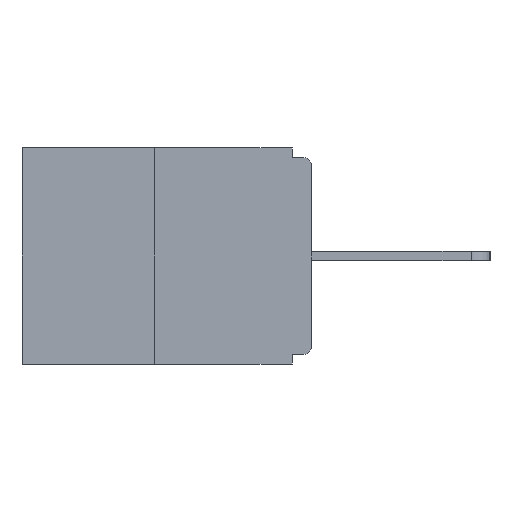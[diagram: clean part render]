
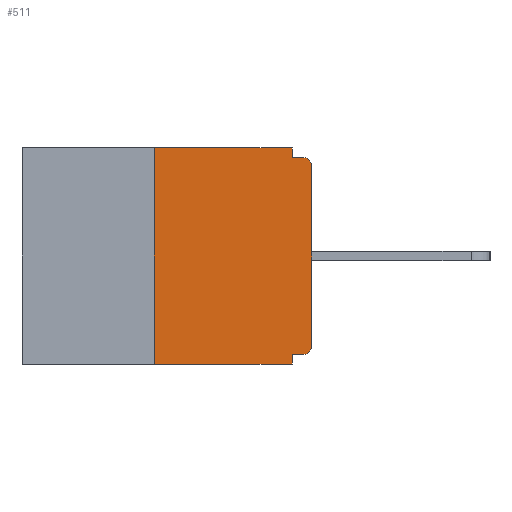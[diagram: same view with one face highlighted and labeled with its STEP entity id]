
A CAD part, left-side view. The second image highlights one B-rep face of the part: STEP entity #511.
In plain terms, the highlighted planar face has unit normal (-1, 0, 0).
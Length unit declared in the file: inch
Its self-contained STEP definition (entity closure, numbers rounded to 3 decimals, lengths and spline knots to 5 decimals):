
#488 = VECTOR ( 'NONE', #17203, 39.37008 ) ;
#509 = DIRECTION ( 'NONE',  ( 0., 0., 1. ) ) ;
#511 = ADVANCED_FACE ( 'NONE', ( #11315 ), #3797, .F. ) ;
#588 = CARTESIAN_POINT ( 'NONE',  ( 0., 0., 0. ) ) ;
#759 = DIRECTION ( 'NONE',  ( 1., 0., 0. ) ) ;
#874 = DIRECTION ( 'NONE',  ( 0., -1., 0. ) ) ;
#1120 = EDGE_LOOP ( 'NONE', ( #9245, #10424, #9022, #7291, #12049, #1280, #16525, #9086, #8726, #9004 ) ) ;
#1280 = ORIENTED_EDGE ( 'NONE', *, *, #3385, .T. ) ;
#1300 = VECTOR ( 'NONE', #509, 39.37008 ) ;
#1647 = VERTEX_POINT ( 'NONE', #1875 ) ;
#1843 = DIRECTION ( 'NONE',  ( 0., -1., 0. ) ) ;
#1875 = CARTESIAN_POINT ( 'NONE',  ( 0., 0., -0.03 ) ) ;
#2244 = CARTESIAN_POINT ( 'NONE',  ( 0., 0.25, 0. ) ) ;
#2885 = CARTESIAN_POINT ( 'NONE',  ( 0., 0.015, -0.03 ) ) ;
#2975 = CARTESIAN_POINT ( 'NONE',  ( 0., 0.031, -0.015 ) ) ;
#3385 = EDGE_CURVE ( 'NONE', #7476, #16054, #7079, .T. ) ;
#3548 = EDGE_CURVE ( 'NONE', #16054, #1647, #18411, .T. ) ;
#3797 = PLANE ( 'NONE',  #12862 ) ;
#3869 = LINE ( 'NONE', #6156, #15055 ) ;
#4214 = DIRECTION ( 'NONE',  ( -1., 0., 0. ) ) ;
#4341 = EDGE_CURVE ( 'NONE', #9982, #6168, #6028, .T. ) ;
#4819 = AXIS2_PLACEMENT_3D ( 'NONE', #2885, #10698, #16344 ) ;
#5270 = DIRECTION ( 'NONE',  ( 0., 0., -1. ) ) ;
#5628 = CARTESIAN_POINT ( 'NONE',  ( 0., 0.46, 0. ) ) ;
#6028 = LINE ( 'NONE', #5628, #488 ) ;
#6156 = CARTESIAN_POINT ( 'NONE',  ( 0., 0.031, -0.343 ) ) ;
#6168 = VERTEX_POINT ( 'NONE', #12745 ) ;
#6912 = CARTESIAN_POINT ( 'NONE',  ( 0., 0., -0.328 ) ) ;
#7079 = CIRCLE ( 'NONE', #17907, 0.015 ) ;
#7291 = ORIENTED_EDGE ( 'NONE', *, *, #10679, .F. ) ;
#7476 = VERTEX_POINT ( 'NONE', #11408 ) ;
#7525 = VECTOR ( 'NONE', #9132, 39.37008 ) ;
#8483 = CARTESIAN_POINT ( 'NONE',  ( 0., 0.015, -0.015 ) ) ;
#8532 = EDGE_CURVE ( 'NONE', #17141, #13712, #15683, .T. ) ;
#8726 = ORIENTED_EDGE ( 'NONE', *, *, #8532, .F. ) ;
#9004 = ORIENTED_EDGE ( 'NONE', *, *, #15616, .F. ) ;
#9014 = VERTEX_POINT ( 'NONE', #18674 ) ;
#9022 = ORIENTED_EDGE ( 'NONE', *, *, #18537, .T. ) ;
#9086 = ORIENTED_EDGE ( 'NONE', *, *, #9792, .T. ) ;
#9132 = DIRECTION ( 'NONE',  ( 0., 0., 1. ) ) ;
#9245 = ORIENTED_EDGE ( 'NONE', *, *, #4341, .F. ) ;
#9532 = CARTESIAN_POINT ( 'NONE',  ( 0., 0., -0.015 ) ) ;
#9620 = VERTEX_POINT ( 'NONE', #10843 ) ;
#9792 = EDGE_CURVE ( 'NONE', #1647, #13712, #12235, .T. ) ;
#9847 = DIRECTION ( 'NONE',  ( 0., 1., 0. ) ) ;
#9982 = VERTEX_POINT ( 'NONE', #13771 ) ;
#10038 = CARTESIAN_POINT ( 'NONE',  ( 0., 0.015, -0.313 ) ) ;
#10086 = EDGE_CURVE ( 'NONE', #7476, #9014, #17677, .T. ) ;
#10424 = ORIENTED_EDGE ( 'NONE', *, *, #15927, .F. ) ;
#10634 = CARTESIAN_POINT ( 'NONE',  ( 0., 0.031, 0. ) ) ;
#10679 = EDGE_CURVE ( 'NONE', #9014, #9620, #3869, .T. ) ;
#10698 = DIRECTION ( 'NONE',  ( -1., 0., 0. ) ) ;
#10843 = CARTESIAN_POINT ( 'NONE',  ( 0., 0.031, -0.343 ) ) ;
#11090 = LINE ( 'NONE', #13755, #13369 ) ;
#11148 = CARTESIAN_POINT ( 'NONE',  ( 0., 0.46, 0. ) ) ;
#11315 = FACE_OUTER_BOUND ( 'NONE', #1120, .T. ) ;
#11408 = CARTESIAN_POINT ( 'NONE',  ( 0., 0.015, -0.328 ) ) ;
#12049 = ORIENTED_EDGE ( 'NONE', *, *, #10086, .F. ) ;
#12235 = CIRCLE ( 'NONE', #4819, 0.015 ) ;
#12745 = CARTESIAN_POINT ( 'NONE',  ( 0., 0.031, 0. ) ) ;
#12840 = CARTESIAN_POINT ( 'NONE',  ( 0., 0., -0.313 ) ) ;
#12862 = AXIS2_PLACEMENT_3D ( 'NONE', #11148, #759, #5270 ) ;
#13346 = CARTESIAN_POINT ( 'NONE',  ( 0., 0.25, -0.343 ) ) ;
#13369 = VECTOR ( 'NONE', #1843, 39.37008 ) ;
#13557 = DIRECTION ( 'NONE',  ( 0., 0., -1. ) ) ;
#13562 = DIRECTION ( 'NONE',  ( 0., 0., -1. ) ) ;
#13712 = VERTEX_POINT ( 'NONE', #8483 ) ;
#13755 = CARTESIAN_POINT ( 'NONE',  ( 0., 0.46, -0.343 ) ) ;
#13771 = CARTESIAN_POINT ( 'NONE',  ( 0., 0.25, 0. ) ) ;
#14294 = VERTEX_POINT ( 'NONE', #13346 ) ;
#14429 = DIRECTION ( 'NONE',  ( 0., 0., -1. ) ) ;
#15055 = VECTOR ( 'NONE', #13557, 39.37008 ) ;
#15240 = VECTOR ( 'NONE', #874, 39.37008 ) ;
#15616 = EDGE_CURVE ( 'NONE', #6168, #17141, #17524, .T. ) ;
#15683 = LINE ( 'NONE', #9532, #15240 ) ;
#15927 = EDGE_CURVE ( 'NONE', #14294, #9982, #17958, .T. ) ;
#16054 = VERTEX_POINT ( 'NONE', #12840 ) ;
#16344 = DIRECTION ( 'NONE',  ( 0., 0., -1. ) ) ;
#16525 = ORIENTED_EDGE ( 'NONE', *, *, #3548, .T. ) ;
#17141 = VERTEX_POINT ( 'NONE', #2975 ) ;
#17203 = DIRECTION ( 'NONE',  ( 0., -1., 0. ) ) ;
#17524 = LINE ( 'NONE', #10634, #18416 ) ;
#17677 = LINE ( 'NONE', #6912, #18559 ) ;
#17907 = AXIS2_PLACEMENT_3D ( 'NONE', #10038, #4214, #14429 ) ;
#17958 = LINE ( 'NONE', #2244, #1300 ) ;
#18411 = LINE ( 'NONE', #588, #7525 ) ;
#18416 = VECTOR ( 'NONE', #13562, 39.37008 ) ;
#18537 = EDGE_CURVE ( 'NONE', #14294, #9620, #11090, .T. ) ;
#18559 = VECTOR ( 'NONE', #9847, 39.37008 ) ;
#18674 = CARTESIAN_POINT ( 'NONE',  ( 0., 0.031, -0.328 ) ) ;
